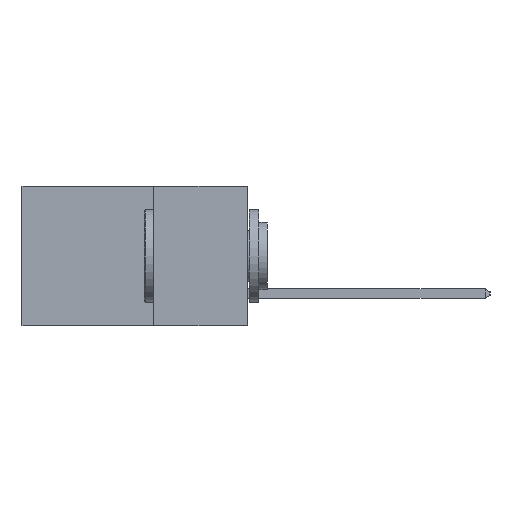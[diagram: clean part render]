
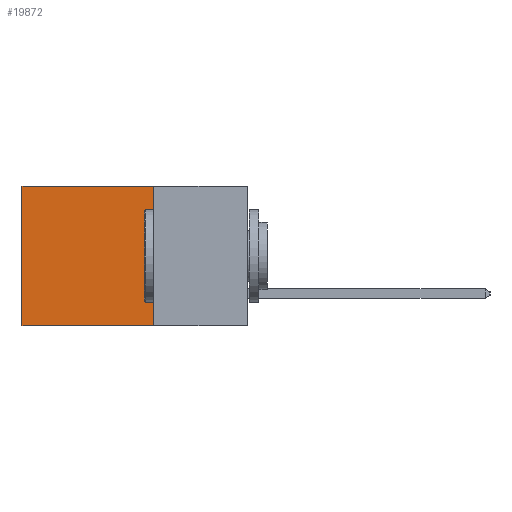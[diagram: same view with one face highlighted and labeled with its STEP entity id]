
A CAD part, left-side view. The second image highlights one B-rep face of the part: STEP entity #19872.
In plain terms, the highlighted planar face has unit normal (-1, 0, 0).
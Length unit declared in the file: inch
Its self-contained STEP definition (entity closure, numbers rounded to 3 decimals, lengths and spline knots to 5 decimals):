
#222 = CARTESIAN_POINT ( 'NONE',  ( 0.2615, 0.25, -0.37 ) ) ;
#641 = VERTEX_POINT ( 'NONE', #2638 ) ;
#2430 = CARTESIAN_POINT ( 'NONE',  ( 0.2615, 0.6, -0.37 ) ) ;
#2638 = CARTESIAN_POINT ( 'NONE',  ( 0.2615, 0.6, 0. ) ) ;
#2790 = VECTOR ( 'NONE', #19743, 39.37008 ) ;
#2952 = VECTOR ( 'NONE', #18602, 39.37008 ) ;
#3427 = ORIENTED_EDGE ( 'NONE', *, *, #19496, .T. ) ;
#3701 = EDGE_CURVE ( 'NONE', #7100, #6678, #7563, .T. ) ;
#3733 = DIRECTION ( 'NONE',  ( 0., 0., -1. ) ) ;
#5814 = VERTEX_POINT ( 'NONE', #12944 ) ;
#6678 = VERTEX_POINT ( 'NONE', #2430 ) ;
#6977 = VECTOR ( 'NONE', #7644, 39.37008 ) ;
#7098 = CARTESIAN_POINT ( 'NONE',  ( 0.2615, 0.25, 0. ) ) ;
#7100 = VERTEX_POINT ( 'NONE', #14885 ) ;
#7563 = LINE ( 'NONE', #19843, #2790 ) ;
#7644 = DIRECTION ( 'NONE',  ( 0., 1., 0. ) ) ;
#7939 = EDGE_CURVE ( 'NONE', #5814, #641, #11662, .T. ) ;
#10773 = PLANE ( 'NONE',  #20939 ) ;
#10816 = DIRECTION ( 'NONE',  ( 0., 0., -1. ) ) ;
#11048 = CARTESIAN_POINT ( 'NONE',  ( 0.2615, 0.25, -0.37 ) ) ;
#11581 = ORIENTED_EDGE ( 'NONE', *, *, #3701, .F. ) ;
#11662 = LINE ( 'NONE', #7098, #6977 ) ;
#12944 = CARTESIAN_POINT ( 'NONE',  ( 0.2615, 0.25, 0. ) ) ;
#14348 = DIRECTION ( 'NONE',  ( 1., 0., 0. ) ) ;
#14357 = EDGE_CURVE ( 'NONE', #5814, #7100, #20125, .T. ) ;
#14462 = VECTOR ( 'NONE', #10816, 39.37008 ) ;
#14650 = ORIENTED_EDGE ( 'NONE', *, *, #7939, .T. ) ;
#14885 = CARTESIAN_POINT ( 'NONE',  ( 0.2615, 0.25, -0.37 ) ) ;
#16901 = CARTESIAN_POINT ( 'NONE',  ( 0.2615, 0.6, -0.37 ) ) ;
#17085 = LINE ( 'NONE', #16901, #2952 ) ;
#17808 = EDGE_LOOP ( 'NONE', ( #3427, #11581, #18134, #14650 ) ) ;
#18123 = FACE_OUTER_BOUND ( 'NONE', #17808, .T. ) ;
#18134 = ORIENTED_EDGE ( 'NONE', *, *, #14357, .F. ) ;
#18602 = DIRECTION ( 'NONE',  ( 0., 0., -1. ) ) ;
#19496 = EDGE_CURVE ( 'NONE', #641, #6678, #17085, .T. ) ;
#19743 = DIRECTION ( 'NONE',  ( 0., 1., 0. ) ) ;
#19843 = CARTESIAN_POINT ( 'NONE',  ( 0.2615, 0.25, -0.37 ) ) ;
#19872 = ADVANCED_FACE ( 'NONE', ( #18123 ), #10773, .F. ) ;
#20125 = LINE ( 'NONE', #11048, #14462 ) ;
#20939 = AXIS2_PLACEMENT_3D ( 'NONE', #222, #14348, #3733 ) ;
